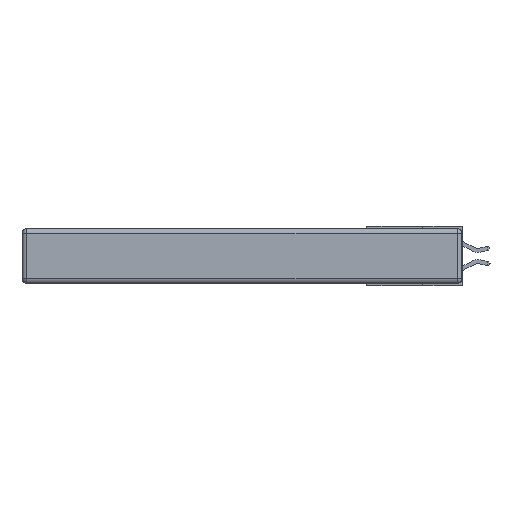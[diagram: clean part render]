
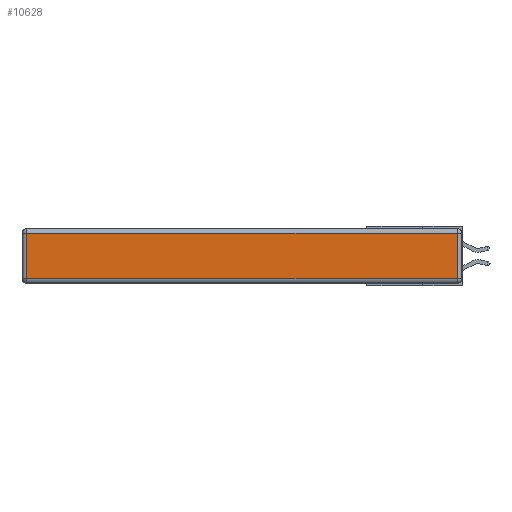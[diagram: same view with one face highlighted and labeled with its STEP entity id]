
A CAD part, left-side view. The second image highlights one B-rep face of the part: STEP entity #10628.
In plain terms, the highlighted planar face has unit normal (-1, 0, 0).
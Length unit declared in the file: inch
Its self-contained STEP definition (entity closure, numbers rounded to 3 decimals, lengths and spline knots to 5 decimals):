
#1015 = EDGE_CURVE ( 'NONE', #33798, #30157, #25710, .T. ) ;
#1819 = CARTESIAN_POINT ( 'NONE',  ( 0., 0., -0.313 ) ) ;
#2627 = CARTESIAN_POINT ( 'NONE',  ( 0., 0.03, -0.03 ) ) ;
#3871 = CARTESIAN_POINT ( 'NONE',  ( 0., 2.72, -0.313 ) ) ;
#4236 = CARTESIAN_POINT ( 'NONE',  ( 0., 2.75, -0.03 ) ) ;
#4393 = DIRECTION ( 'NONE',  ( 0., -1., 0. ) ) ;
#4930 = VERTEX_POINT ( 'NONE', #2627 ) ;
#5628 = LINE ( 'NONE', #13721, #9866 ) ;
#6961 = DIRECTION ( 'NONE',  ( 0., 1., 0. ) ) ;
#7098 = VECTOR ( 'NONE', #4393, 39.37008 ) ;
#7606 = LINE ( 'NONE', #10322, #26619 ) ;
#8403 = ORIENTED_EDGE ( 'NONE', *, *, #21309, .T. ) ;
#8547 = FACE_OUTER_BOUND ( 'NONE', #23737, .T. ) ;
#9533 = ORIENTED_EDGE ( 'NONE', *, *, #14820, .T. ) ;
#9866 = VECTOR ( 'NONE', #29581, 39.37008 ) ;
#10322 = CARTESIAN_POINT ( 'NONE',  ( 0., 0.03, -0.343 ) ) ;
#10628 = ADVANCED_FACE ( 'NONE', ( #8547 ), #18610, .T. ) ;
#13265 = AXIS2_PLACEMENT_3D ( 'NONE', #18716, #13392, #32309 ) ;
#13341 = EDGE_CURVE ( 'NONE', #4930, #15514, #20243, .T. ) ;
#13392 = DIRECTION ( 'NONE',  ( -1., 0., 0. ) ) ;
#13721 = CARTESIAN_POINT ( 'NONE',  ( 0., 2.72, -0.343 ) ) ;
#14820 = EDGE_CURVE ( 'NONE', #15514, #33798, #5628, .T. ) ;
#15514 = VERTEX_POINT ( 'NONE', #27889 ) ;
#15540 = ORIENTED_EDGE ( 'NONE', *, *, #1015, .T. ) ;
#18610 = PLANE ( 'NONE',  #13265 ) ;
#18716 = CARTESIAN_POINT ( 'NONE',  ( 0., 0., -0.343 ) ) ;
#19139 = ORIENTED_EDGE ( 'NONE', *, *, #13341, .T. ) ;
#20243 = LINE ( 'NONE', #4236, #28675 ) ;
#21309 = EDGE_CURVE ( 'NONE', #30157, #4930, #7606, .T. ) ;
#23737 = EDGE_LOOP ( 'NONE', ( #15540, #8403, #19139, #9533 ) ) ;
#25710 = LINE ( 'NONE', #1819, #7098 ) ;
#26619 = VECTOR ( 'NONE', #31459, 39.37008 ) ;
#27777 = CARTESIAN_POINT ( 'NONE',  ( 0., 0.03, -0.313 ) ) ;
#27889 = CARTESIAN_POINT ( 'NONE',  ( 0., 2.72, -0.03 ) ) ;
#28675 = VECTOR ( 'NONE', #6961, 39.37008 ) ;
#29581 = DIRECTION ( 'NONE',  ( 0., 0., -1. ) ) ;
#30157 = VERTEX_POINT ( 'NONE', #27777 ) ;
#31459 = DIRECTION ( 'NONE',  ( 0., 0., 1. ) ) ;
#32309 = DIRECTION ( 'NONE',  ( 0., 0., 1. ) ) ;
#33798 = VERTEX_POINT ( 'NONE', #3871 ) ;
